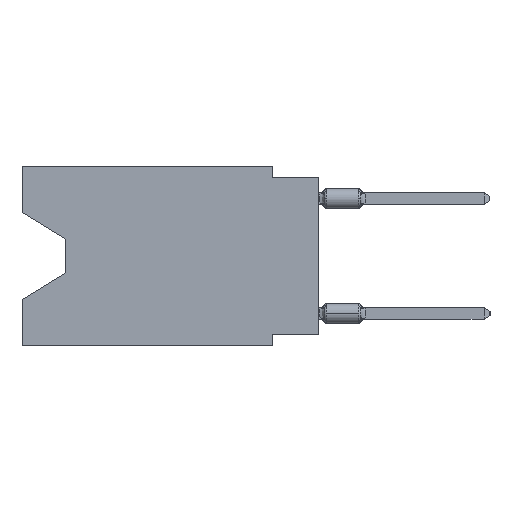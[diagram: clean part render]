
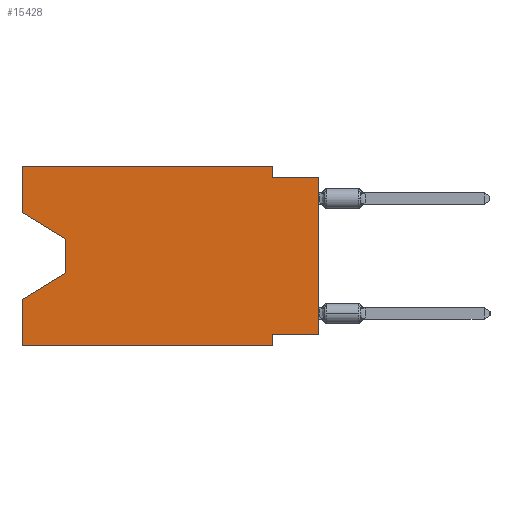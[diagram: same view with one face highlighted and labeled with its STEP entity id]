
A CAD part, left-side view. The second image highlights one B-rep face of the part: STEP entity #15428.
In plain terms, the highlighted planar face has unit normal (-1, 0, 0).
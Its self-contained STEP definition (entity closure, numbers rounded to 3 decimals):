
#421 = CARTESIAN_POINT ( 'NONE',  ( 0., 16.383, 0. ) ) ;
#923 = VECTOR ( 'NONE', #16717, 1000. ) ;
#1804 = LINE ( 'NONE', #8233, #22354 ) ;
#2000 = CARTESIAN_POINT ( 'NONE',  ( 0., 0., -9.271 ) ) ;
#2426 = EDGE_CURVE ( 'NONE', #31748, #22359, #19988, .T. ) ;
#2830 = EDGE_CURVE ( 'NONE', #22359, #9228, #16097, .T. ) ;
#3673 = DIRECTION ( 'NONE',  ( 0., 0., 1. ) ) ;
#4544 = CARTESIAN_POINT ( 'NONE',  ( 0., 16.383, -9.906 ) ) ;
#4847 = CARTESIAN_POINT ( 'NONE',  ( 0., 2.54, -9.906 ) ) ;
#5297 = ORIENTED_EDGE ( 'NONE', *, *, #2830, .F. ) ;
#5354 = CARTESIAN_POINT ( 'NONE',  ( 0., 16.383, -2.546 ) ) ;
#5910 = DIRECTION ( 'NONE',  ( 1., 0., 0. ) ) ;
#6167 = CARTESIAN_POINT ( 'NONE',  ( 0., 2.54, -9.271 ) ) ;
#6282 = VECTOR ( 'NONE', #36919, 1000. ) ;
#6494 = EDGE_CURVE ( 'NONE', #26108, #40695, #20853, .T. ) ;
#7145 = VERTEX_POINT ( 'NONE', #6167 ) ;
#7513 = LINE ( 'NONE', #10116, #31878 ) ;
#8133 = CARTESIAN_POINT ( 'NONE',  ( 0., 13.97, -5.893 ) ) ;
#8233 = CARTESIAN_POINT ( 'NONE',  ( 0., 0., -9.271 ) ) ;
#8996 = VERTEX_POINT ( 'NONE', #2000 ) ;
#9228 = VERTEX_POINT ( 'NONE', #19971 ) ;
#9681 = CARTESIAN_POINT ( 'NONE',  ( 0., 16.383, 0. ) ) ;
#10116 = CARTESIAN_POINT ( 'NONE',  ( 0., 0., 0. ) ) ;
#10735 = CARTESIAN_POINT ( 'NONE',  ( 0., 13.97, -4.013 ) ) ;
#10774 = CARTESIAN_POINT ( 'NONE',  ( 0., 2.54, -9.906 ) ) ;
#10866 = VECTOR ( 'NONE', #23599, 1000. ) ;
#12203 = LINE ( 'NONE', #8133, #39513 ) ;
#12574 = EDGE_CURVE ( 'NONE', #9228, #24005, #30502, .T. ) ;
#12751 = FACE_OUTER_BOUND ( 'NONE', #39702, .T. ) ;
#12853 = LINE ( 'NONE', #22959, #923 ) ;
#13160 = CARTESIAN_POINT ( 'NONE',  ( 0., 16.383, 0. ) ) ;
#13825 = ORIENTED_EDGE ( 'NONE', *, *, #20689, .F. ) ;
#13946 = DIRECTION ( 'NONE',  ( 0., 0., -1. ) ) ;
#14217 = ORIENTED_EDGE ( 'NONE', *, *, #31797, .T. ) ;
#14245 = CARTESIAN_POINT ( 'NONE',  ( 0., 0., -0.635 ) ) ;
#15331 = EDGE_CURVE ( 'NONE', #26108, #20657, #39343, .T. ) ;
#15428 = ADVANCED_FACE ( 'NONE', ( #12751 ), #19827, .F. ) ;
#16097 = LINE ( 'NONE', #421, #10866 ) ;
#16717 = DIRECTION ( 'NONE',  ( 0., -0.855, -0.519 ) ) ;
#17307 = VECTOR ( 'NONE', #23712, 1000. ) ;
#17715 = VERTEX_POINT ( 'NONE', #39381 ) ;
#18186 = CARTESIAN_POINT ( 'NONE',  ( 0., 16.383, 0. ) ) ;
#18452 = VECTOR ( 'NONE', #30814, 1000. ) ;
#18570 = VECTOR ( 'NONE', #13946, 1000. ) ;
#18995 = DIRECTION ( 'NONE',  ( 0., 0., -1. ) ) ;
#19827 = PLANE ( 'NONE',  #28461 ) ;
#19971 = CARTESIAN_POINT ( 'NONE',  ( 0., 2.54, 0. ) ) ;
#19988 = LINE ( 'NONE', #9681, #26713 ) ;
#20144 = ORIENTED_EDGE ( 'NONE', *, *, #12574, .F. ) ;
#20180 = LINE ( 'NONE', #10735, #18570 ) ;
#20657 = VERTEX_POINT ( 'NONE', #33126 ) ;
#20689 = EDGE_CURVE ( 'NONE', #24005, #17715, #40208, .T. ) ;
#20853 = LINE ( 'NONE', #4544, #6282 ) ;
#21339 = DIRECTION ( 'NONE',  ( 0., 1., 0. ) ) ;
#21803 = CARTESIAN_POINT ( 'NONE',  ( 0., 2.54, -0.635 ) ) ;
#22219 = CARTESIAN_POINT ( 'NONE',  ( 0., 16.383, 0. ) ) ;
#22354 = VECTOR ( 'NONE', #21339, 1000. ) ;
#22359 = VERTEX_POINT ( 'NONE', #18186 ) ;
#22715 = VECTOR ( 'NONE', #40353, 1000. ) ;
#22959 = CARTESIAN_POINT ( 'NONE',  ( 0., 16.383, -2.546 ) ) ;
#23284 = VERTEX_POINT ( 'NONE', #27742 ) ;
#23450 = EDGE_CURVE ( 'NONE', #8996, #17715, #7513, .T. ) ;
#23599 = DIRECTION ( 'NONE',  ( 0., -1., 0. ) ) ;
#23648 = DIRECTION ( 'NONE',  ( 0., 0., 1. ) ) ;
#23712 = DIRECTION ( 'NONE',  ( 0., -1., 0. ) ) ;
#24005 = VERTEX_POINT ( 'NONE', #21803 ) ;
#24644 = ORIENTED_EDGE ( 'NONE', *, *, #26038, .F. ) ;
#25663 = ORIENTED_EDGE ( 'NONE', *, *, #23450, .T. ) ;
#26038 = EDGE_CURVE ( 'NONE', #8996, #7145, #1804, .T. ) ;
#26108 = VERTEX_POINT ( 'NONE', #27990 ) ;
#26689 = ORIENTED_EDGE ( 'NONE', *, *, #6494, .T. ) ;
#26713 = VECTOR ( 'NONE', #3673, 1000. ) ;
#27280 = CARTESIAN_POINT ( 'NONE',  ( 0., 2.54, 0. ) ) ;
#27406 = ORIENTED_EDGE ( 'NONE', *, *, #36045, .F. ) ;
#27426 = VERTEX_POINT ( 'NONE', #35053 ) ;
#27742 = CARTESIAN_POINT ( 'NONE',  ( 0., 13.97, -5.893 ) ) ;
#27990 = CARTESIAN_POINT ( 'NONE',  ( 0., 16.383, -9.906 ) ) ;
#28461 = AXIS2_PLACEMENT_3D ( 'NONE', #22219, #5910, #18995 ) ;
#29589 = ORIENTED_EDGE ( 'NONE', *, *, #2426, .F. ) ;
#30502 = LINE ( 'NONE', #27280, #22715 ) ;
#30814 = DIRECTION ( 'NONE',  ( 0., 0., -1. ) ) ;
#30884 = DIRECTION ( 'NONE',  ( 0., 0.855, -0.519 ) ) ;
#31583 = ORIENTED_EDGE ( 'NONE', *, *, #15331, .F. ) ;
#31748 = VERTEX_POINT ( 'NONE', #5354 ) ;
#31797 = EDGE_CURVE ( 'NONE', #23284, #20657, #12203, .T. ) ;
#31878 = VECTOR ( 'NONE', #23648, 1000. ) ;
#32465 = ORIENTED_EDGE ( 'NONE', *, *, #38430, .T. ) ;
#32512 = ORIENTED_EDGE ( 'NONE', *, *, #40834, .T. ) ;
#33126 = CARTESIAN_POINT ( 'NONE',  ( 0., 16.383, -7.36 ) ) ;
#35053 = CARTESIAN_POINT ( 'NONE',  ( 0., 13.97, -4.013 ) ) ;
#36045 = EDGE_CURVE ( 'NONE', #7145, #40695, #40684, .T. ) ;
#36919 = DIRECTION ( 'NONE',  ( 0., -1., 0. ) ) ;
#38430 = EDGE_CURVE ( 'NONE', #27426, #23284, #20180, .T. ) ;
#39119 = DIRECTION ( 'NONE',  ( 0., 0., 1. ) ) ;
#39343 = LINE ( 'NONE', #13160, #42162 ) ;
#39381 = CARTESIAN_POINT ( 'NONE',  ( 0., 0., -0.635 ) ) ;
#39513 = VECTOR ( 'NONE', #30884, 1000. ) ;
#39702 = EDGE_LOOP ( 'NONE', ( #32512, #32465, #14217, #31583, #26689, #27406, #24644, #25663, #13825, #20144, #5297, #29589 ) ) ;
#40208 = LINE ( 'NONE', #14245, #17307 ) ;
#40353 = DIRECTION ( 'NONE',  ( 0., 0., -1. ) ) ;
#40684 = LINE ( 'NONE', #4847, #18452 ) ;
#40695 = VERTEX_POINT ( 'NONE', #10774 ) ;
#40834 = EDGE_CURVE ( 'NONE', #31748, #27426, #12853, .T. ) ;
#42162 = VECTOR ( 'NONE', #39119, 1000. ) ;
